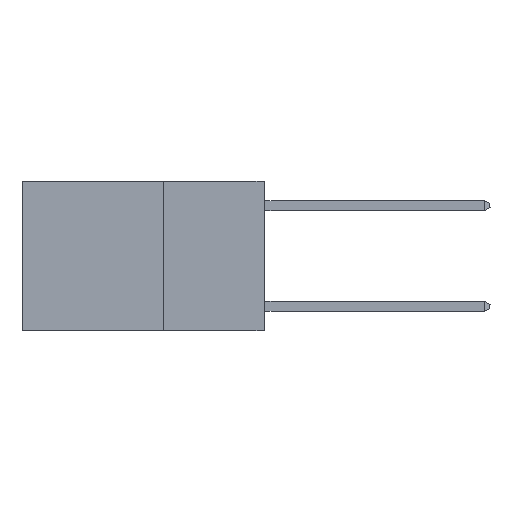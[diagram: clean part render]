
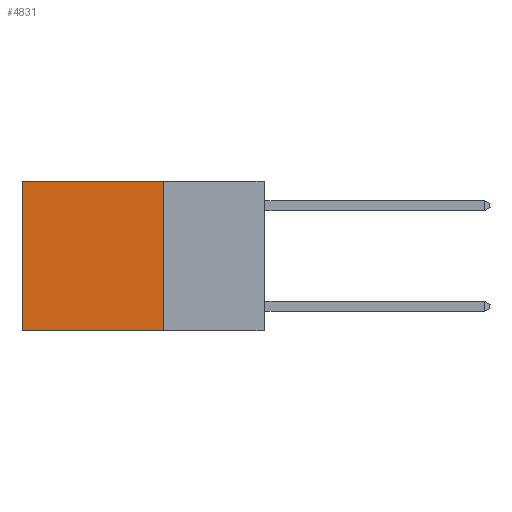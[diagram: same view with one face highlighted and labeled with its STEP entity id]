
A CAD part, left-side view. The second image highlights one B-rep face of the part: STEP entity #4831.
In plain terms, the highlighted face is planar.
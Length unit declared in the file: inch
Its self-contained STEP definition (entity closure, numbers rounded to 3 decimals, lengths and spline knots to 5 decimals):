
#2138 = LINE ( 'NONE', #17014, #4092 ) ;
#2189 = AXIS2_PLACEMENT_3D ( 'NONE', #14279, #16588, #3472 ) ;
#3239 = EDGE_CURVE ( 'NONE', #24986, #16103, #8830, .T. ) ;
#3472 = DIRECTION ( 'NONE',  ( 0., 0., -1. ) ) ;
#4092 = VECTOR ( 'NONE', #17692, 39.37008 ) ;
#4334 = LINE ( 'NONE', #19459, #7237 ) ;
#4361 = CARTESIAN_POINT ( 'NONE',  ( 0.2625, 0.6, 0. ) ) ;
#4805 = CARTESIAN_POINT ( 'NONE',  ( 0.2625, 0.25, -0.37 ) ) ;
#4831 = ADVANCED_FACE ( 'NONE', ( #10108 ), #21468, .F. ) ;
#4983 = EDGE_CURVE ( 'NONE', #9776, #16103, #4334, .T. ) ;
#5129 = CARTESIAN_POINT ( 'NONE',  ( 0.2625, 0.25, 0. ) ) ;
#5822 = ORIENTED_EDGE ( 'NONE', *, *, #8722, .F. ) ;
#6166 = EDGE_LOOP ( 'NONE', ( #10668, #10528, #5822, #22254 ) ) ;
#7237 = VECTOR ( 'NONE', #28215, 39.37008 ) ;
#8722 = EDGE_CURVE ( 'NONE', #20264, #9776, #2138, .T. ) ;
#8830 = LINE ( 'NONE', #4361, #17771 ) ;
#9508 = CARTESIAN_POINT ( 'NONE',  ( 0.2625, 0.6, -0.37 ) ) ;
#9774 = CARTESIAN_POINT ( 'NONE',  ( 0.2625, 0.6, 0. ) ) ;
#9776 = VERTEX_POINT ( 'NONE', #4805 ) ;
#10108 = FACE_OUTER_BOUND ( 'NONE', #6166, .T. ) ;
#10528 = ORIENTED_EDGE ( 'NONE', *, *, #4983, .F. ) ;
#10668 = ORIENTED_EDGE ( 'NONE', *, *, #3239, .T. ) ;
#13143 = DIRECTION ( 'NONE',  ( 0., 0., -1. ) ) ;
#14279 = CARTESIAN_POINT ( 'NONE',  ( 0.2625, 0.25, 0. ) ) ;
#14990 = LINE ( 'NONE', #25496, #17966 ) ;
#16103 = VERTEX_POINT ( 'NONE', #9508 ) ;
#16588 = DIRECTION ( 'NONE',  ( 1., 0., 0. ) ) ;
#17014 = CARTESIAN_POINT ( 'NONE',  ( 0.2625, 0.25, 0. ) ) ;
#17692 = DIRECTION ( 'NONE',  ( 0., 0., -1. ) ) ;
#17771 = VECTOR ( 'NONE', #13143, 39.37008 ) ;
#17966 = VECTOR ( 'NONE', #21175, 39.37008 ) ;
#19459 = CARTESIAN_POINT ( 'NONE',  ( 0.2625, 0.25, -0.37 ) ) ;
#20264 = VERTEX_POINT ( 'NONE', #5129 ) ;
#21175 = DIRECTION ( 'NONE',  ( 0., 1., 0. ) ) ;
#21468 = PLANE ( 'NONE',  #2189 ) ;
#21493 = EDGE_CURVE ( 'NONE', #20264, #24986, #14990, .T. ) ;
#22254 = ORIENTED_EDGE ( 'NONE', *, *, #21493, .T. ) ;
#24986 = VERTEX_POINT ( 'NONE', #9774 ) ;
#25496 = CARTESIAN_POINT ( 'NONE',  ( 0.2625, 0.25, 0. ) ) ;
#28215 = DIRECTION ( 'NONE',  ( 0., 1., 0. ) ) ;
